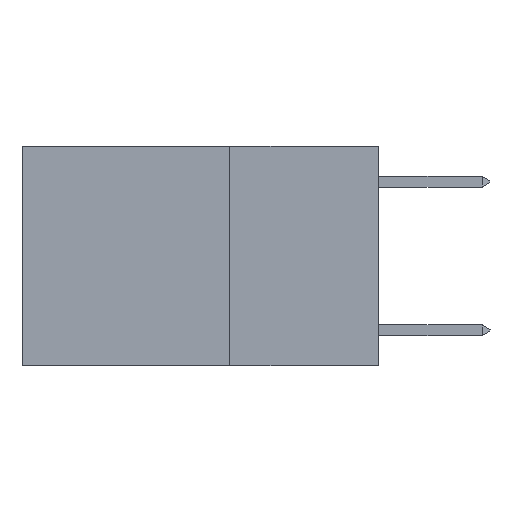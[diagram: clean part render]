
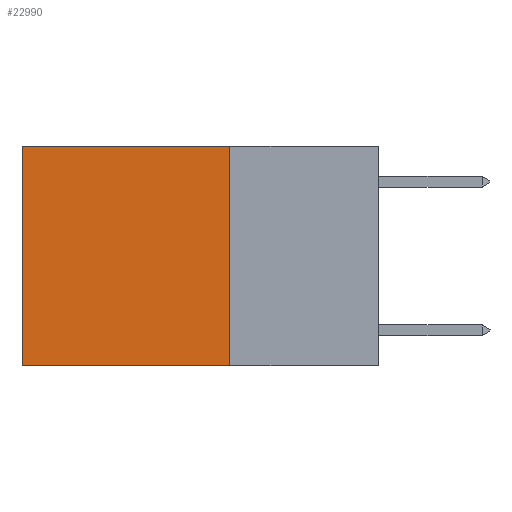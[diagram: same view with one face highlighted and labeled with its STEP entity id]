
A CAD part, left-side view. The second image highlights one B-rep face of the part: STEP entity #22990.
In plain terms, the highlighted planar face has unit normal (-1, 0, 0).
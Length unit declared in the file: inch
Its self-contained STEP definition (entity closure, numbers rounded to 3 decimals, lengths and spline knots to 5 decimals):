
#288 = CARTESIAN_POINT ( 'NONE',  ( 0.2625, 0.25, 0. ) ) ;
#739 = CARTESIAN_POINT ( 'NONE',  ( 0.2625, 0.25, -0.37 ) ) ;
#1854 = ORIENTED_EDGE ( 'NONE', *, *, #24905, .F. ) ;
#1966 = EDGE_LOOP ( 'NONE', ( #17024, #1854, #22711, #18460 ) ) ;
#2303 = DIRECTION ( 'NONE',  ( 1., 0., 0. ) ) ;
#2504 = VECTOR ( 'NONE', #3701, 39.37008 ) ;
#2711 = DIRECTION ( 'NONE',  ( 0., 1., 0. ) ) ;
#2714 = LINE ( 'NONE', #5710, #2504 ) ;
#3559 = LINE ( 'NONE', #11067, #19234 ) ;
#3701 = DIRECTION ( 'NONE',  ( 0., 1., 0. ) ) ;
#4813 = FACE_OUTER_BOUND ( 'NONE', #1966, .T. ) ;
#5710 = CARTESIAN_POINT ( 'NONE',  ( 0.2625, 0.25, 0. ) ) ;
#6594 = VECTOR ( 'NONE', #2711, 39.37008 ) ;
#8762 = VERTEX_POINT ( 'NONE', #13510 ) ;
#9360 = DIRECTION ( 'NONE',  ( 0., 0., -1. ) ) ;
#9824 = CARTESIAN_POINT ( 'NONE',  ( 0.2625, 0.6, -0.37 ) ) ;
#11067 = CARTESIAN_POINT ( 'NONE',  ( 0.2625, 0.6, 0. ) ) ;
#11184 = CARTESIAN_POINT ( 'NONE',  ( 0.2625, 0.25, -0.37 ) ) ;
#11233 = CARTESIAN_POINT ( 'NONE',  ( 0.2625, 0.25, 0. ) ) ;
#12237 = PLANE ( 'NONE',  #22253 ) ;
#13510 = CARTESIAN_POINT ( 'NONE',  ( 0.2625, 0.6, 0. ) ) ;
#15406 = EDGE_CURVE ( 'NONE', #20487, #21691, #20277, .T. ) ;
#16156 = DIRECTION ( 'NONE',  ( 0., 0., -1. ) ) ;
#17024 = ORIENTED_EDGE ( 'NONE', *, *, #22319, .T. ) ;
#17668 = LINE ( 'NONE', #739, #6594 ) ;
#17955 = EDGE_CURVE ( 'NONE', #20487, #8762, #2714, .T. ) ;
#18460 = ORIENTED_EDGE ( 'NONE', *, *, #17955, .T. ) ;
#19234 = VECTOR ( 'NONE', #24253, 39.37008 ) ;
#20144 = VECTOR ( 'NONE', #9360, 39.37008 ) ;
#20277 = LINE ( 'NONE', #24493, #20144 ) ;
#20487 = VERTEX_POINT ( 'NONE', #11233 ) ;
#21691 = VERTEX_POINT ( 'NONE', #11184 ) ;
#22253 = AXIS2_PLACEMENT_3D ( 'NONE', #288, #2303, #16156 ) ;
#22319 = EDGE_CURVE ( 'NONE', #8762, #23472, #3559, .T. ) ;
#22711 = ORIENTED_EDGE ( 'NONE', *, *, #15406, .F. ) ;
#22990 = ADVANCED_FACE ( 'NONE', ( #4813 ), #12237, .F. ) ;
#23472 = VERTEX_POINT ( 'NONE', #9824 ) ;
#24253 = DIRECTION ( 'NONE',  ( 0., 0., -1. ) ) ;
#24493 = CARTESIAN_POINT ( 'NONE',  ( 0.2625, 0.25, 0. ) ) ;
#24905 = EDGE_CURVE ( 'NONE', #21691, #23472, #17668, .T. ) ;
